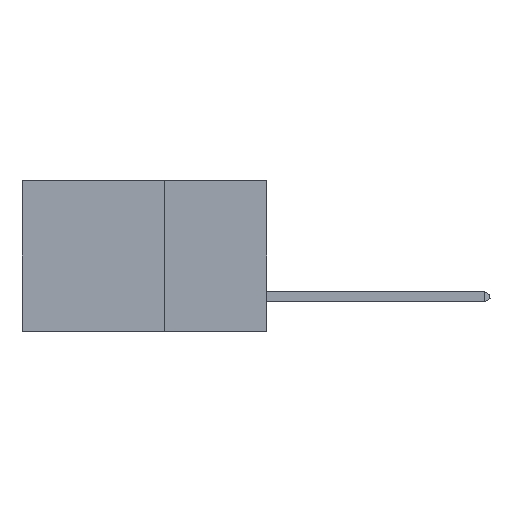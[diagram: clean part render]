
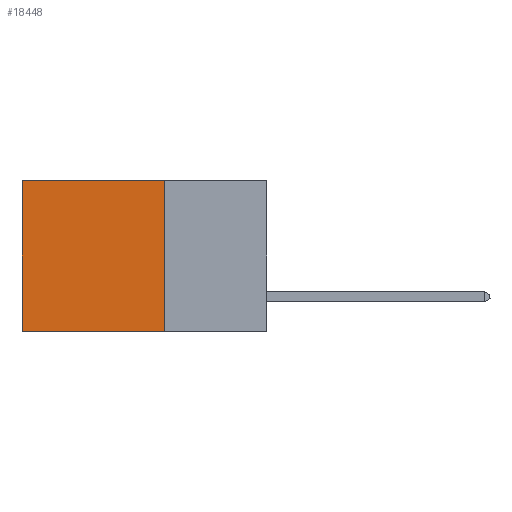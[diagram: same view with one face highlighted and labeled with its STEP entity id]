
A CAD part, left-side view. The second image highlights one B-rep face of the part: STEP entity #18448.
In plain terms, the highlighted planar face has unit normal (-1, 0, 0).
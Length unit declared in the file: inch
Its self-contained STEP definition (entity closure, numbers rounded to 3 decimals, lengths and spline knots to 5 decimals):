
#2117 = VERTEX_POINT ( 'NONE', #18603 ) ;
#3350 = EDGE_CURVE ( 'NONE', #25788, #2117, #25116, .T. ) ;
#3662 = AXIS2_PLACEMENT_3D ( 'NONE', #20861, #7000, #21038 ) ;
#4272 = VECTOR ( 'NONE', #18945, 39.37008 ) ;
#4928 = CARTESIAN_POINT ( 'NONE',  ( 0.2875, 0.6, 0. ) ) ;
#4980 = PLANE ( 'NONE',  #3662 ) ;
#6101 = CARTESIAN_POINT ( 'NONE',  ( 0.2875, 0.25, 0. ) ) ;
#6299 = VERTEX_POINT ( 'NONE', #24879 ) ;
#6702 = ORIENTED_EDGE ( 'NONE', *, *, #17713, .F. ) ;
#7000 = DIRECTION ( 'NONE',  ( 1., 0., 0. ) ) ;
#7522 = ORIENTED_EDGE ( 'NONE', *, *, #19497, .T. ) ;
#9607 = VERTEX_POINT ( 'NONE', #4928 ) ;
#10050 = CARTESIAN_POINT ( 'NONE',  ( 0.2875, 0.6, 0. ) ) ;
#11620 = DIRECTION ( 'NONE',  ( 0., 0., -1. ) ) ;
#14798 = CARTESIAN_POINT ( 'NONE',  ( 0.2875, 0.25, 0. ) ) ;
#15354 = ORIENTED_EDGE ( 'NONE', *, *, #3350, .F. ) ;
#15451 = VECTOR ( 'NONE', #18230, 39.37008 ) ;
#16510 = LINE ( 'NONE', #14798, #4272 ) ;
#17713 = EDGE_CURVE ( 'NONE', #2117, #6299, #24500, .T. ) ;
#18011 = CARTESIAN_POINT ( 'NONE',  ( 0.2875, 0.25, -0.37 ) ) ;
#18087 = ORIENTED_EDGE ( 'NONE', *, *, #25186, .T. ) ;
#18230 = DIRECTION ( 'NONE',  ( 0., 0., -1. ) ) ;
#18448 = ADVANCED_FACE ( 'NONE', ( #18491 ), #4980, .F. ) ;
#18491 = FACE_OUTER_BOUND ( 'NONE', #25984, .T. ) ;
#18603 = CARTESIAN_POINT ( 'NONE',  ( 0.2875, 0.25, -0.37 ) ) ;
#18863 = VECTOR ( 'NONE', #11620, 39.37008 ) ;
#18945 = DIRECTION ( 'NONE',  ( 0., 1., 0. ) ) ;
#19497 = EDGE_CURVE ( 'NONE', #25788, #9607, #16510, .T. ) ;
#20219 = CARTESIAN_POINT ( 'NONE',  ( 0.2875, 0.25, 0. ) ) ;
#20861 = CARTESIAN_POINT ( 'NONE',  ( 0.2875, 0.25, 0. ) ) ;
#21038 = DIRECTION ( 'NONE',  ( 0., 0., -1. ) ) ;
#21812 = DIRECTION ( 'NONE',  ( 0., 1., 0. ) ) ;
#22067 = LINE ( 'NONE', #10050, #15451 ) ;
#22627 = VECTOR ( 'NONE', #21812, 39.37008 ) ;
#24500 = LINE ( 'NONE', #18011, #22627 ) ;
#24879 = CARTESIAN_POINT ( 'NONE',  ( 0.2875, 0.6, -0.37 ) ) ;
#25116 = LINE ( 'NONE', #6101, #18863 ) ;
#25186 = EDGE_CURVE ( 'NONE', #9607, #6299, #22067, .T. ) ;
#25788 = VERTEX_POINT ( 'NONE', #20219 ) ;
#25984 = EDGE_LOOP ( 'NONE', ( #18087, #6702, #15354, #7522 ) ) ;
